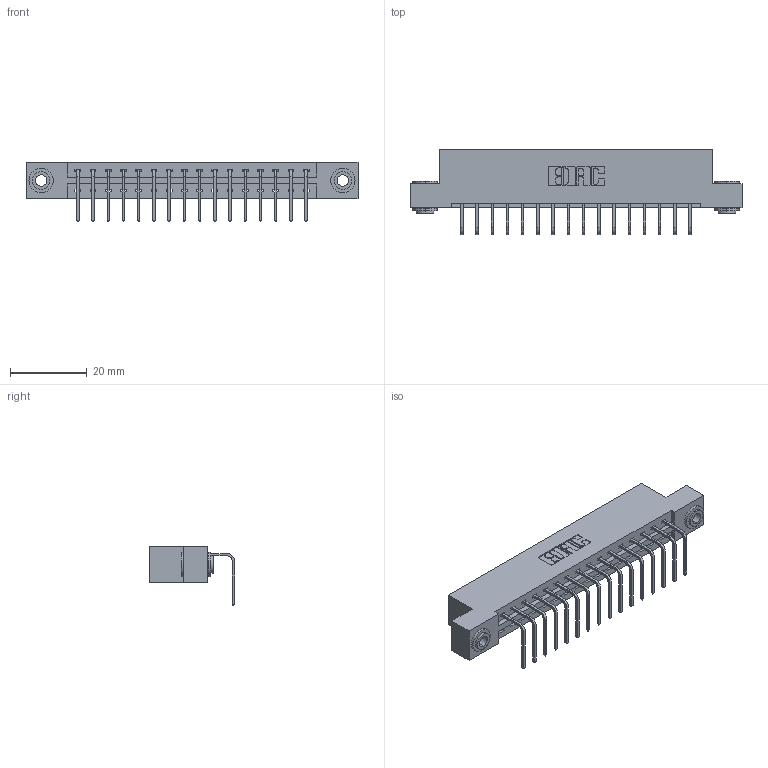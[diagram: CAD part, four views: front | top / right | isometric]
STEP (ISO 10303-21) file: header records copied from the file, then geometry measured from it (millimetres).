
FILE_DESCRIPTION (( 'STEP AP203' ), '1' );
FILE_NAME ('337-016-558-103.STEP', '2018-08-04T20:27:44', ( '' ), ( '' ), 'SwSTEP 2.0', 'SolidWorks 2016', '' );
FILE_SCHEMA (( 'CONFIG_CONTROL_DESIGN' ));
Length unit declared in the file: inch
Products named in the file (4): 337 Part_Flush Mounting Lugs - 0.156 Dia-TH; 345-292-001_558 Tail - 2; 345-250-002_345-250-002-102; 337-016-558-103
Assembly tree (19 placements, depth 2):
  337-016-558-103
    337 Part_Flush Mounting Lugs - 0.156 Dia-TH
    345-292-001_558 Tail - 2  x16
    345-250-002_345-250-002-102  x2
Bounding box: 86.41 x 22.17 x 15.37 mm (x, y, z)
Volume: 8728.3 mm3; surface area: 9435.3 mm2
Topology: 19 solids, 19 shells, 1176 faces, 3491 edges, 2302 vertices
Faces by surface type: plane 848, cylinder 320, cone 8
Entity records: 15990 total; most frequent: CARTESIAN_POINT 2761, ORIENTED_EDGE 2706, DIRECTION 2411, EDGE_CURVE 1353, VECTOR 1201, LINE 1201, VERTEX_POINT 898, AXIS2_PLACEMENT_3D 605
